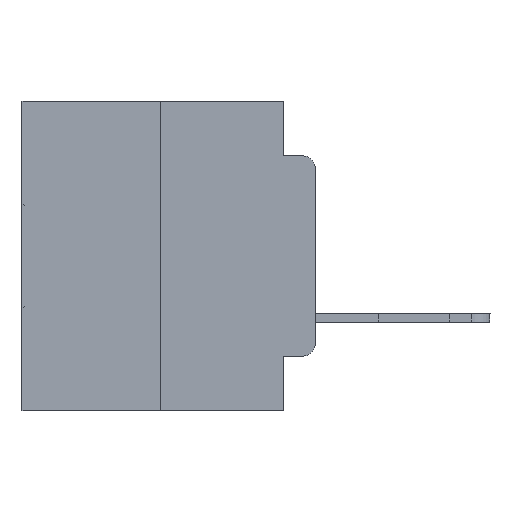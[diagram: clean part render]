
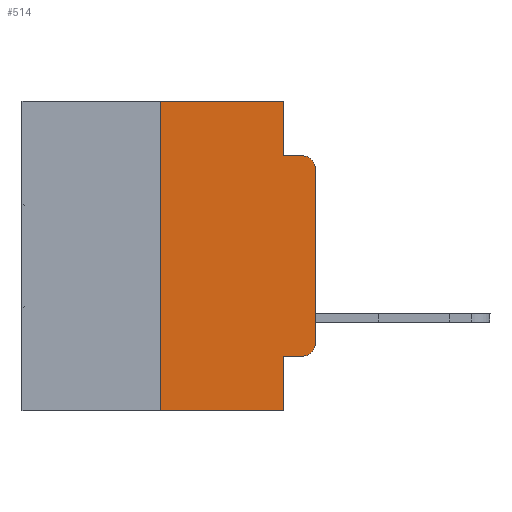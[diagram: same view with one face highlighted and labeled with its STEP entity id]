
A CAD part, left-side view. The second image highlights one B-rep face of the part: STEP entity #514.
In plain terms, the highlighted planar face has unit normal (-1, 0, 0).
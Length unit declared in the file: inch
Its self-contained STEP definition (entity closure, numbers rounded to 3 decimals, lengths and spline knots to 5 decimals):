
#415 = LINE ( 'NONE', #13813, #8017 ) ;
#514 = ADVANCED_FACE ( 'NONE', ( #13069 ), #1805, .F. ) ;
#674 = CIRCLE ( 'NONE', #17005, 0.02 ) ;
#1805 = PLANE ( 'NONE',  #18783 ) ;
#1989 = DIRECTION ( 'NONE',  ( -1., 0., 0. ) ) ;
#2255 = EDGE_CURVE ( 'NONE', #25635, #14779, #26079, .T. ) ;
#3201 = EDGE_CURVE ( 'NONE', #15357, #11014, #27421, .T. ) ;
#3511 = CARTESIAN_POINT ( 'NONE',  ( 0., 0.051, -0.0885 ) ) ;
#4054 = DIRECTION ( 'NONE',  ( 1., 0., 0. ) ) ;
#4063 = LINE ( 'NONE', #26499, #14423 ) ;
#5457 = CIRCLE ( 'NONE', #21014, 0.02 ) ;
#6403 = CARTESIAN_POINT ( 'NONE',  ( 0., 0., -0.1085 ) ) ;
#6669 = ORIENTED_EDGE ( 'NONE', *, *, #22364, .T. ) ;
#7262 = DIRECTION ( 'NONE',  ( 0., 0., -1. ) ) ;
#7825 = DIRECTION ( 'NONE',  ( -1., 0., 0. ) ) ;
#7916 = LINE ( 'NONE', #3511, #19353 ) ;
#7980 = VECTOR ( 'NONE', #28298, 39.37008 ) ;
#8017 = VECTOR ( 'NONE', #18275, 39.37008 ) ;
#8167 = CARTESIAN_POINT ( 'NONE',  ( 0., 0., 0. ) ) ;
#8418 = CARTESIAN_POINT ( 'NONE',  ( 0., 0.25, 0. ) ) ;
#8458 = LINE ( 'NONE', #27205, #9833 ) ;
#8514 = EDGE_CURVE ( 'NONE', #16190, #19374, #23326, .T. ) ;
#8618 = VERTEX_POINT ( 'NONE', #8958 ) ;
#8958 = CARTESIAN_POINT ( 'NONE',  ( 0., 0.02, -0.0885 ) ) ;
#8975 = ORIENTED_EDGE ( 'NONE', *, *, #2255, .F. ) ;
#9307 = ORIENTED_EDGE ( 'NONE', *, *, #26604, .F. ) ;
#9444 = EDGE_LOOP ( 'NONE', ( #10337, #12209, #26175, #9307, #20116, #14212, #24315, #8975, #6669, #23950 ) ) ;
#9599 = EDGE_CURVE ( 'NONE', #11014, #25317, #415, .T. ) ;
#9833 = VECTOR ( 'NONE', #13894, 39.37008 ) ;
#9902 = DIRECTION ( 'NONE',  ( 0., -1., 0. ) ) ;
#10337 = ORIENTED_EDGE ( 'NONE', *, *, #8514, .T. ) ;
#10859 = DIRECTION ( 'NONE',  ( 0., -1., 0. ) ) ;
#10877 = VECTOR ( 'NONE', #7262, 39.37008 ) ;
#10956 = EDGE_CURVE ( 'NONE', #19374, #8618, #5457, .T. ) ;
#11014 = VERTEX_POINT ( 'NONE', #17129 ) ;
#11111 = LINE ( 'NONE', #21647, #7980 ) ;
#11743 = CARTESIAN_POINT ( 'NONE',  ( 0., 0., -0.3915 ) ) ;
#12209 = ORIENTED_EDGE ( 'NONE', *, *, #10956, .T. ) ;
#13069 = FACE_OUTER_BOUND ( 'NONE', #9444, .T. ) ;
#13813 = CARTESIAN_POINT ( 'NONE',  ( 0., 0.473, 0. ) ) ;
#13894 = DIRECTION ( 'NONE',  ( 0., 0., -1. ) ) ;
#14212 = ORIENTED_EDGE ( 'NONE', *, *, #3201, .F. ) ;
#14421 = EDGE_CURVE ( 'NONE', #16096, #16190, #674, .T. ) ;
#14423 = VECTOR ( 'NONE', #10859, 39.37008 ) ;
#14779 = VERTEX_POINT ( 'NONE', #17105 ) ;
#15122 = CARTESIAN_POINT ( 'NONE',  ( 0., 0.051, -0.4115 ) ) ;
#15357 = VERTEX_POINT ( 'NONE', #27590 ) ;
#16096 = VERTEX_POINT ( 'NONE', #24224 ) ;
#16097 = DIRECTION ( 'NONE',  ( 0., 0., -1. ) ) ;
#16190 = VERTEX_POINT ( 'NONE', #11743 ) ;
#17005 = AXIS2_PLACEMENT_3D ( 'NONE', #22197, #1989, #16097 ) ;
#17105 = CARTESIAN_POINT ( 'NONE',  ( 0., 0.051, -0.5 ) ) ;
#17129 = CARTESIAN_POINT ( 'NONE',  ( 0., 0.25, 0. ) ) ;
#17498 = EDGE_CURVE ( 'NONE', #27116, #8618, #7916, .T. ) ;
#18013 = CARTESIAN_POINT ( 'NONE',  ( 0., 0.051, 0. ) ) ;
#18275 = DIRECTION ( 'NONE',  ( 0., -1., 0. ) ) ;
#18783 = AXIS2_PLACEMENT_3D ( 'NONE', #21922, #4054, #21729 ) ;
#19353 = VECTOR ( 'NONE', #9902, 39.37008 ) ;
#19374 = VERTEX_POINT ( 'NONE', #6403 ) ;
#20116 = ORIENTED_EDGE ( 'NONE', *, *, #9599, .F. ) ;
#20455 = CARTESIAN_POINT ( 'NONE',  ( 0., 0.051, -0.0885 ) ) ;
#20696 = CARTESIAN_POINT ( 'NONE',  ( 0., 0.02, -0.1085 ) ) ;
#20979 = DIRECTION ( 'NONE',  ( 0., 0., -1. ) ) ;
#21014 = AXIS2_PLACEMENT_3D ( 'NONE', #20696, #7825, #20979 ) ;
#21647 = CARTESIAN_POINT ( 'NONE',  ( 0., 0.051, -0.4115 ) ) ;
#21729 = DIRECTION ( 'NONE',  ( 0., 0., -1. ) ) ;
#21922 = CARTESIAN_POINT ( 'NONE',  ( 0., 0.473, 0. ) ) ;
#22197 = CARTESIAN_POINT ( 'NONE',  ( 0., 0.02, -0.3915 ) ) ;
#22364 = EDGE_CURVE ( 'NONE', #25635, #16096, #11111, .T. ) ;
#22586 = VECTOR ( 'NONE', #23849, 39.37008 ) ;
#23326 = LINE ( 'NONE', #8167, #25729 ) ;
#23616 = DIRECTION ( 'NONE',  ( 0., 0., 1. ) ) ;
#23849 = DIRECTION ( 'NONE',  ( 0., 0., 1. ) ) ;
#23950 = ORIENTED_EDGE ( 'NONE', *, *, #14421, .T. ) ;
#24224 = CARTESIAN_POINT ( 'NONE',  ( 0., 0.02, -0.4115 ) ) ;
#24315 = ORIENTED_EDGE ( 'NONE', *, *, #25167, .T. ) ;
#24922 = CARTESIAN_POINT ( 'NONE',  ( 0., 0.051, 0. ) ) ;
#25167 = EDGE_CURVE ( 'NONE', #15357, #14779, #4063, .T. ) ;
#25317 = VERTEX_POINT ( 'NONE', #18013 ) ;
#25635 = VERTEX_POINT ( 'NONE', #15122 ) ;
#25729 = VECTOR ( 'NONE', #23616, 39.37008 ) ;
#26079 = LINE ( 'NONE', #24922, #10877 ) ;
#26175 = ORIENTED_EDGE ( 'NONE', *, *, #17498, .F. ) ;
#26499 = CARTESIAN_POINT ( 'NONE',  ( 0., 0.473, -0.5 ) ) ;
#26604 = EDGE_CURVE ( 'NONE', #25317, #27116, #8458, .T. ) ;
#27116 = VERTEX_POINT ( 'NONE', #20455 ) ;
#27205 = CARTESIAN_POINT ( 'NONE',  ( 0., 0.051, 0. ) ) ;
#27421 = LINE ( 'NONE', #8418, #22586 ) ;
#27590 = CARTESIAN_POINT ( 'NONE',  ( 0., 0.25, -0.5 ) ) ;
#28298 = DIRECTION ( 'NONE',  ( 0., -1., 0. ) ) ;
